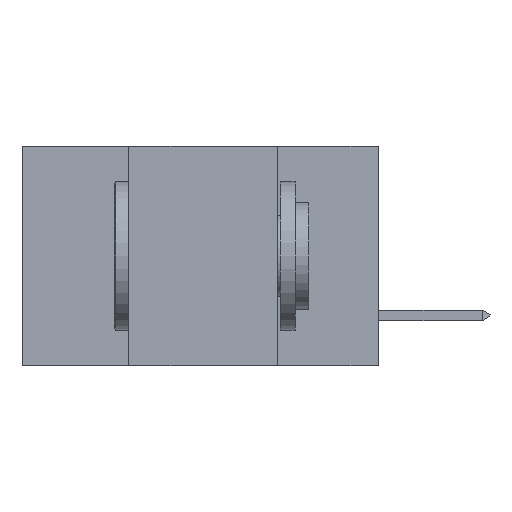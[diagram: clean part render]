
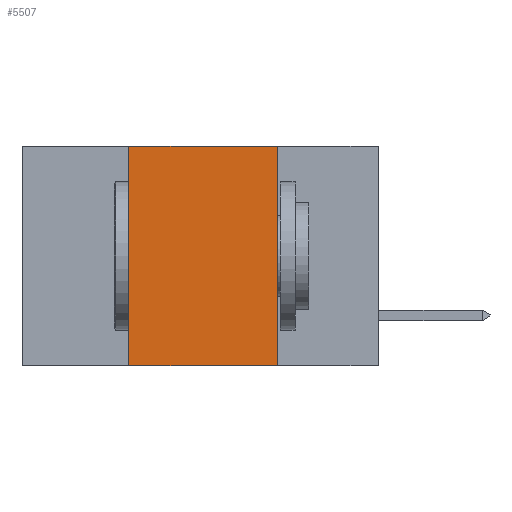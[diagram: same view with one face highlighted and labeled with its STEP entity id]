
A CAD part, left-side view. The second image highlights one B-rep face of the part: STEP entity #5507.
In plain terms, the highlighted planar face has unit normal (-1, 0, 0).
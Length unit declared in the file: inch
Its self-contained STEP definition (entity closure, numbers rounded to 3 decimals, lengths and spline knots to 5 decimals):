
#282 = CARTESIAN_POINT ( 'NONE',  ( 0., 0.42, -0.37 ) ) ;
#2262 = LINE ( 'NONE', #12018, #3563 ) ;
#2452 = DIRECTION ( 'NONE',  ( 0., -1., 0. ) ) ;
#2614 = FACE_OUTER_BOUND ( 'NONE', #7100, .T. ) ;
#3179 = EDGE_CURVE ( 'NONE', #7830, #11927, #12209, .T. ) ;
#3230 = DIRECTION ( 'NONE',  ( 0., 0., 1. ) ) ;
#3563 = VECTOR ( 'NONE', #2452, 39.37008 ) ;
#4163 = VECTOR ( 'NONE', #6319, 39.37008 ) ;
#5287 = CARTESIAN_POINT ( 'NONE',  ( 0., 0.17, -0.37 ) ) ;
#5378 = CARTESIAN_POINT ( 'NONE',  ( 0., 0.6, 0. ) ) ;
#5422 = CARTESIAN_POINT ( 'NONE',  ( 0., 0.17, -0.37 ) ) ;
#5507 = ADVANCED_FACE ( 'NONE', ( #2614 ), #6540, .F. ) ;
#5755 = VECTOR ( 'NONE', #9299, 39.37008 ) ;
#6319 = DIRECTION ( 'NONE',  ( 0., -1., 0. ) ) ;
#6540 = PLANE ( 'NONE',  #11048 ) ;
#6651 = ORIENTED_EDGE ( 'NONE', *, *, #3179, .F. ) ;
#7100 = EDGE_LOOP ( 'NONE', ( #6651, #8047, #7353, #11961 ) ) ;
#7353 = ORIENTED_EDGE ( 'NONE', *, *, #11379, .F. ) ;
#7688 = EDGE_CURVE ( 'NONE', #7857, #7830, #8143, .T. ) ;
#7830 = VERTEX_POINT ( 'NONE', #8531 ) ;
#7857 = VERTEX_POINT ( 'NONE', #8832 ) ;
#8047 = ORIENTED_EDGE ( 'NONE', *, *, #7688, .F. ) ;
#8143 = LINE ( 'NONE', #12012, #4163 ) ;
#8531 = CARTESIAN_POINT ( 'NONE',  ( 0., 0.17, 0. ) ) ;
#8832 = CARTESIAN_POINT ( 'NONE',  ( 0., 0.42, 0. ) ) ;
#9013 = EDGE_CURVE ( 'NONE', #9764, #11927, #2262, .T. ) ;
#9299 = DIRECTION ( 'NONE',  ( 0., 0., -1. ) ) ;
#9585 = LINE ( 'NONE', #282, #12352 ) ;
#9764 = VERTEX_POINT ( 'NONE', #10262 ) ;
#10201 = DIRECTION ( 'NONE',  ( 0., 0., -1. ) ) ;
#10262 = CARTESIAN_POINT ( 'NONE',  ( 0., 0.42, -0.37 ) ) ;
#11048 = AXIS2_PLACEMENT_3D ( 'NONE', #5378, #12107, #10201 ) ;
#11379 = EDGE_CURVE ( 'NONE', #9764, #7857, #9585, .T. ) ;
#11927 = VERTEX_POINT ( 'NONE', #5287 ) ;
#11961 = ORIENTED_EDGE ( 'NONE', *, *, #9013, .T. ) ;
#12012 = CARTESIAN_POINT ( 'NONE',  ( 0., 0.6, 0. ) ) ;
#12018 = CARTESIAN_POINT ( 'NONE',  ( 0., 0.6, -0.37 ) ) ;
#12107 = DIRECTION ( 'NONE',  ( 1., 0., 0. ) ) ;
#12209 = LINE ( 'NONE', #5422, #5755 ) ;
#12352 = VECTOR ( 'NONE', #3230, 39.37008 ) ;
